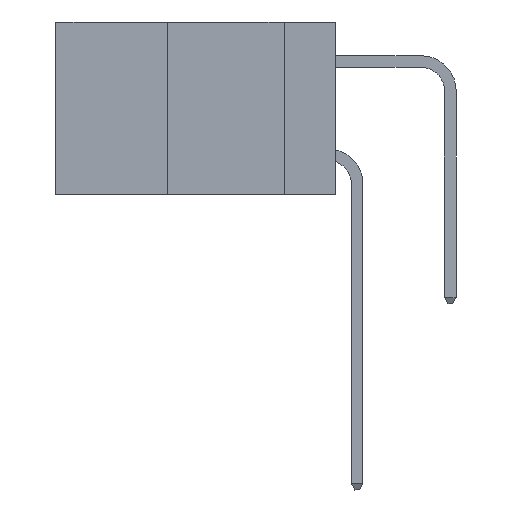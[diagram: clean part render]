
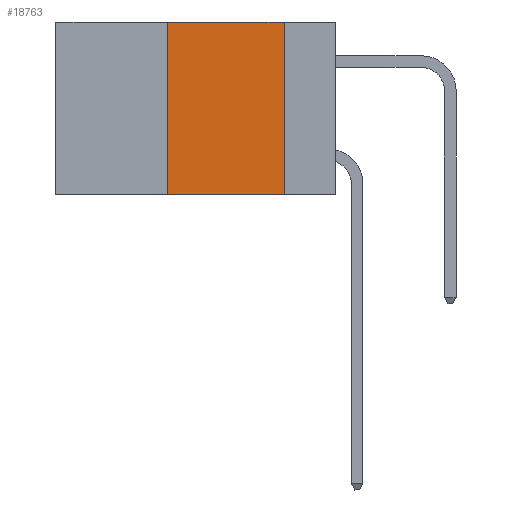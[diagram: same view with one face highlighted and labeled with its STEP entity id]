
A CAD part, left-side view. The second image highlights one B-rep face of the part: STEP entity #18763.
In plain terms, the highlighted planar face has unit normal (-1, 0, 0).
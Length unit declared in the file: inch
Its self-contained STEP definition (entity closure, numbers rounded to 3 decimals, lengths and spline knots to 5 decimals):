
#743 = ORIENTED_EDGE ( 'NONE', *, *, #15293, .T. ) ;
#1027 = CARTESIAN_POINT ( 'NONE',  ( 0., 0.6, -0.37 ) ) ;
#2534 = AXIS2_PLACEMENT_3D ( 'NONE', #6674, #21984, #10578 ) ;
#3079 = DIRECTION ( 'NONE',  ( 0., -1., 0. ) ) ;
#3145 = CARTESIAN_POINT ( 'NONE',  ( 0., 0.36, -0.37 ) ) ;
#3254 = FACE_OUTER_BOUND ( 'NONE', #17652, .T. ) ;
#5375 = VERTEX_POINT ( 'NONE', #24526 ) ;
#6210 = CARTESIAN_POINT ( 'NONE',  ( 0., 0.6, 0. ) ) ;
#6674 = CARTESIAN_POINT ( 'NONE',  ( 0., 0.6, 0. ) ) ;
#7677 = LINE ( 'NONE', #10555, #22301 ) ;
#9134 = CARTESIAN_POINT ( 'NONE',  ( 0., 0.11, 0. ) ) ;
#10555 = CARTESIAN_POINT ( 'NONE',  ( 0., 0.36, 0. ) ) ;
#10578 = DIRECTION ( 'NONE',  ( 0., 0., -1. ) ) ;
#11054 = DIRECTION ( 'NONE',  ( 0., 0., -1. ) ) ;
#11658 = VECTOR ( 'NONE', #3079, 39.37008 ) ;
#11907 = VERTEX_POINT ( 'NONE', #3145 ) ;
#12254 = LINE ( 'NONE', #1027, #11658 ) ;
#12353 = LINE ( 'NONE', #9134, #17493 ) ;
#12521 = DIRECTION ( 'NONE',  ( 0., 0., 1. ) ) ;
#13704 = ORIENTED_EDGE ( 'NONE', *, *, #21431, .F. ) ;
#14080 = VERTEX_POINT ( 'NONE', #18727 ) ;
#14995 = VERTEX_POINT ( 'NONE', #21382 ) ;
#15293 = EDGE_CURVE ( 'NONE', #11907, #14995, #12254, .T. ) ;
#17493 = VECTOR ( 'NONE', #11054, 39.37008 ) ;
#17652 = EDGE_LOOP ( 'NONE', ( #18178, #13704, #23697, #743 ) ) ;
#17796 = DIRECTION ( 'NONE',  ( 0., -1., 0. ) ) ;
#18178 = ORIENTED_EDGE ( 'NONE', *, *, #19563, .F. ) ;
#18727 = CARTESIAN_POINT ( 'NONE',  ( 0., 0.36, 0. ) ) ;
#18763 = ADVANCED_FACE ( 'NONE', ( #3254 ), #20118, .F. ) ;
#18966 = LINE ( 'NONE', #6210, #19564 ) ;
#19563 = EDGE_CURVE ( 'NONE', #5375, #14995, #12353, .T. ) ;
#19564 = VECTOR ( 'NONE', #17796, 39.37008 ) ;
#20118 = PLANE ( 'NONE',  #2534 ) ;
#21382 = CARTESIAN_POINT ( 'NONE',  ( 0., 0.11, -0.37 ) ) ;
#21431 = EDGE_CURVE ( 'NONE', #14080, #5375, #18966, .T. ) ;
#21984 = DIRECTION ( 'NONE',  ( 1., 0., 0. ) ) ;
#22301 = VECTOR ( 'NONE', #12521, 39.37008 ) ;
#23697 = ORIENTED_EDGE ( 'NONE', *, *, #24522, .F. ) ;
#24522 = EDGE_CURVE ( 'NONE', #11907, #14080, #7677, .T. ) ;
#24526 = CARTESIAN_POINT ( 'NONE',  ( 0., 0.11, 0. ) ) ;
